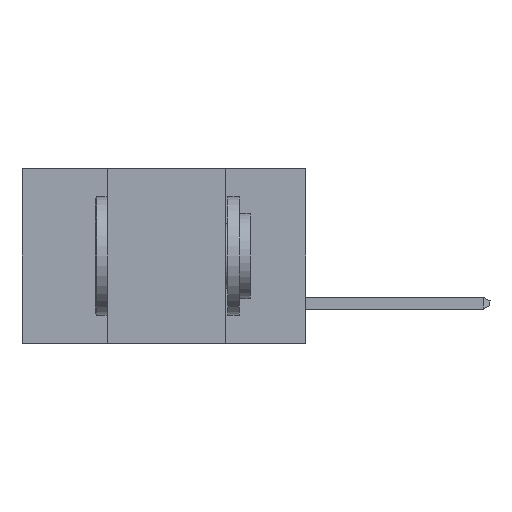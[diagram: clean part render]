
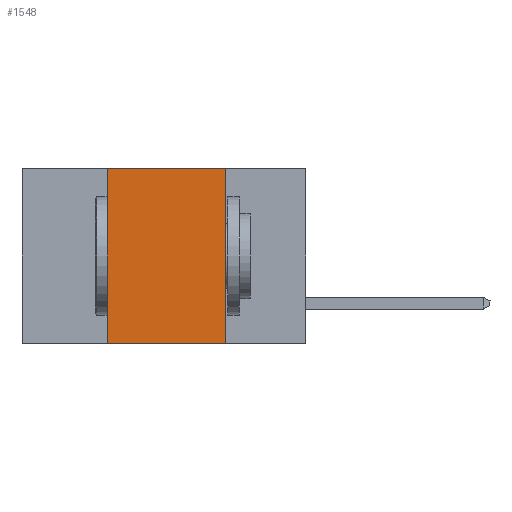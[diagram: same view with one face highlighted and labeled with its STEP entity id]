
A CAD part, left-side view. The second image highlights one B-rep face of the part: STEP entity #1548.
In plain terms, the highlighted planar face has unit normal (-1, 0, 0).
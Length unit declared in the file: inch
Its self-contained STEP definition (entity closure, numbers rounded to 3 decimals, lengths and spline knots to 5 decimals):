
#173 = DIRECTION ( 'NONE',  ( 0., 0., -1. ) ) ;
#680 = LINE ( 'NONE', #3571, #8990 ) ;
#1020 = LINE ( 'NONE', #6081, #8839 ) ;
#1293 = CARTESIAN_POINT ( 'NONE',  ( 0., 0.6, 0. ) ) ;
#1548 = ADVANCED_FACE ( 'NONE', ( #7214 ), #7268, .F. ) ;
#1910 = CARTESIAN_POINT ( 'NONE',  ( 0., 0.17, -0.37 ) ) ;
#2024 = DIRECTION ( 'NONE',  ( 0., 0., -1. ) ) ;
#3222 = ORIENTED_EDGE ( 'NONE', *, *, #3979, .T. ) ;
#3571 = CARTESIAN_POINT ( 'NONE',  ( 0., 0.42, -0.37 ) ) ;
#3979 = EDGE_CURVE ( 'NONE', #6052, #4243, #11323, .T. ) ;
#4243 = VERTEX_POINT ( 'NONE', #1910 ) ;
#5134 = ORIENTED_EDGE ( 'NONE', *, *, #5847, .F. ) ;
#5520 = CARTESIAN_POINT ( 'NONE',  ( 0., 0.17, -0.37 ) ) ;
#5847 = EDGE_CURVE ( 'NONE', #11221, #4243, #10521, .T. ) ;
#5955 = DIRECTION ( 'NONE',  ( 0., -1., 0. ) ) ;
#6052 = VERTEX_POINT ( 'NONE', #7419 ) ;
#6081 = CARTESIAN_POINT ( 'NONE',  ( 0., 0.6, 0. ) ) ;
#6264 = ORIENTED_EDGE ( 'NONE', *, *, #9259, .F. ) ;
#6330 = CARTESIAN_POINT ( 'NONE',  ( 0., 0.6, -0.37 ) ) ;
#7072 = ORIENTED_EDGE ( 'NONE', *, *, #12626, .F. ) ;
#7214 = FACE_OUTER_BOUND ( 'NONE', #9401, .T. ) ;
#7268 = PLANE ( 'NONE',  #7357 ) ;
#7338 = DIRECTION ( 'NONE',  ( 1., 0., 0. ) ) ;
#7357 = AXIS2_PLACEMENT_3D ( 'NONE', #1293, #7338, #173 ) ;
#7419 = CARTESIAN_POINT ( 'NONE',  ( 0., 0.42, -0.37 ) ) ;
#7720 = VERTEX_POINT ( 'NONE', #10160 ) ;
#8839 = VECTOR ( 'NONE', #5955, 39.37008 ) ;
#8990 = VECTOR ( 'NONE', #11792, 39.37008 ) ;
#9259 = EDGE_CURVE ( 'NONE', #6052, #7720, #680, .T. ) ;
#9401 = EDGE_LOOP ( 'NONE', ( #5134, #7072, #6264, #3222 ) ) ;
#10160 = CARTESIAN_POINT ( 'NONE',  ( 0., 0.42, 0. ) ) ;
#10344 = DIRECTION ( 'NONE',  ( 0., -1., 0. ) ) ;
#10521 = LINE ( 'NONE', #5520, #10963 ) ;
#10754 = CARTESIAN_POINT ( 'NONE',  ( 0., 0.17, 0. ) ) ;
#10963 = VECTOR ( 'NONE', #2024, 39.37008 ) ;
#11221 = VERTEX_POINT ( 'NONE', #10754 ) ;
#11323 = LINE ( 'NONE', #6330, #11344 ) ;
#11344 = VECTOR ( 'NONE', #10344, 39.37008 ) ;
#11792 = DIRECTION ( 'NONE',  ( 0., 0., 1. ) ) ;
#12626 = EDGE_CURVE ( 'NONE', #7720, #11221, #1020, .T. ) ;
